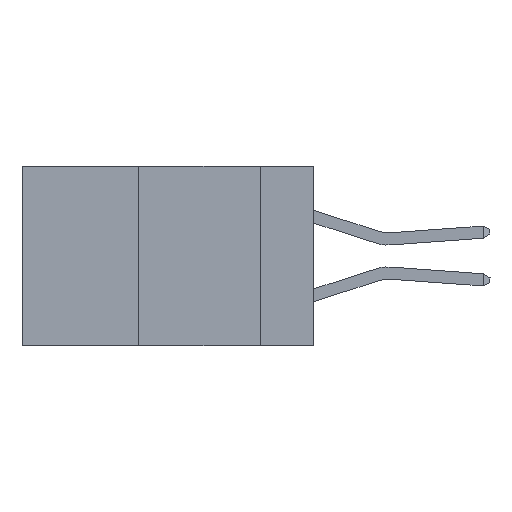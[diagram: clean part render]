
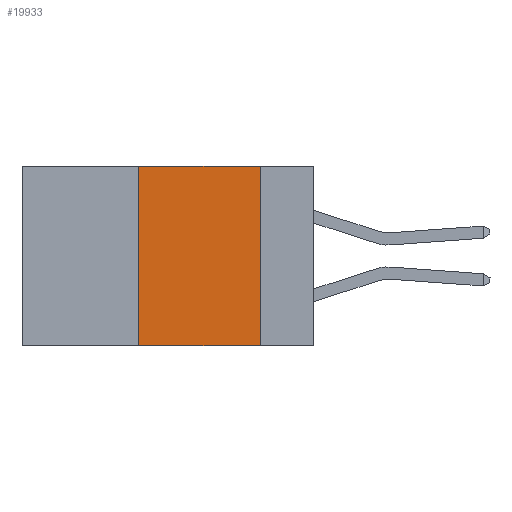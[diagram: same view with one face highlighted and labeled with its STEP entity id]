
A CAD part, left-side view. The second image highlights one B-rep face of the part: STEP entity #19933.
In plain terms, the highlighted planar face has unit normal (-1, 0, 0).
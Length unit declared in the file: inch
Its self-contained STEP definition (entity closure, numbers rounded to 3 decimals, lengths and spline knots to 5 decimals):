
#1115 = EDGE_CURVE ( 'NONE', #11388, #38977, #27689, .T. ) ;
#1775 = CARTESIAN_POINT ( 'NONE',  ( 0., 0.11, 0. ) ) ;
#5516 = EDGE_CURVE ( 'NONE', #11032, #38977, #43043, .T. ) ;
#8334 = EDGE_CURVE ( 'NONE', #14208, #11032, #22542, .T. ) ;
#11032 = VERTEX_POINT ( 'NONE', #27848 ) ;
#11355 = CARTESIAN_POINT ( 'NONE',  ( 0., 0.36, 0. ) ) ;
#11388 = VERTEX_POINT ( 'NONE', #32190 ) ;
#11390 = CARTESIAN_POINT ( 'NONE',  ( 0., 0.6, 0. ) ) ;
#12205 = AXIS2_PLACEMENT_3D ( 'NONE', #28155, #13911, #34840 ) ;
#12234 = EDGE_LOOP ( 'NONE', ( #26278, #28051, #20758, #36174 ) ) ;
#12639 = CARTESIAN_POINT ( 'NONE',  ( 0., 0.11, -0.37 ) ) ;
#13208 = VECTOR ( 'NONE', #29792, 39.37008 ) ;
#13482 = CARTESIAN_POINT ( 'NONE',  ( 0., 0.36, 0. ) ) ;
#13842 = DIRECTION ( 'NONE',  ( 0., -1., 0. ) ) ;
#13911 = DIRECTION ( 'NONE',  ( 1., 0., 0. ) ) ;
#14208 = VERTEX_POINT ( 'NONE', #11355 ) ;
#15048 = DIRECTION ( 'NONE',  ( 0., -1., 0. ) ) ;
#17121 = PLANE ( 'NONE',  #12205 ) ;
#17511 = CARTESIAN_POINT ( 'NONE',  ( 0., 0.6, -0.37 ) ) ;
#19933 = ADVANCED_FACE ( 'NONE', ( #36979 ), #17121, .F. ) ;
#20105 = VECTOR ( 'NONE', #13842, 39.37008 ) ;
#20758 = ORIENTED_EDGE ( 'NONE', *, *, #26771, .F. ) ;
#22542 = LINE ( 'NONE', #11390, #30616 ) ;
#23971 = DIRECTION ( 'NONE',  ( 0., 0., 1. ) ) ;
#26278 = ORIENTED_EDGE ( 'NONE', *, *, #5516, .F. ) ;
#26771 = EDGE_CURVE ( 'NONE', #11388, #14208, #36299, .T. ) ;
#27689 = LINE ( 'NONE', #17511, #20105 ) ;
#27848 = CARTESIAN_POINT ( 'NONE',  ( 0., 0.11, 0. ) ) ;
#28051 = ORIENTED_EDGE ( 'NONE', *, *, #8334, .F. ) ;
#28155 = CARTESIAN_POINT ( 'NONE',  ( 0., 0.6, 0. ) ) ;
#29792 = DIRECTION ( 'NONE',  ( 0., 0., -1. ) ) ;
#30616 = VECTOR ( 'NONE', #15048, 39.37008 ) ;
#32190 = CARTESIAN_POINT ( 'NONE',  ( 0., 0.36, -0.37 ) ) ;
#34840 = DIRECTION ( 'NONE',  ( 0., 0., -1. ) ) ;
#36174 = ORIENTED_EDGE ( 'NONE', *, *, #1115, .T. ) ;
#36299 = LINE ( 'NONE', #13482, #40074 ) ;
#36979 = FACE_OUTER_BOUND ( 'NONE', #12234, .T. ) ;
#38977 = VERTEX_POINT ( 'NONE', #12639 ) ;
#40074 = VECTOR ( 'NONE', #23971, 39.37008 ) ;
#43043 = LINE ( 'NONE', #1775, #13208 ) ;
